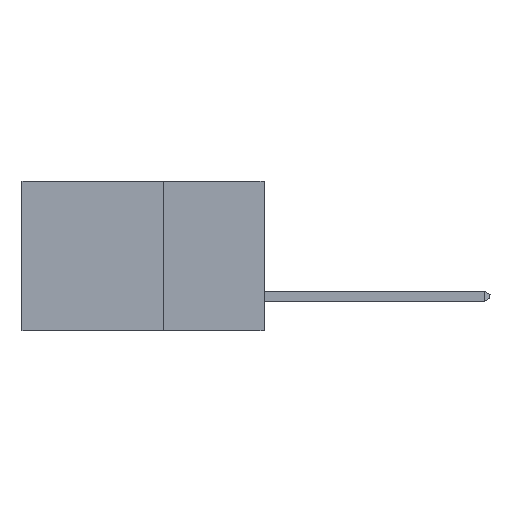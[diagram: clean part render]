
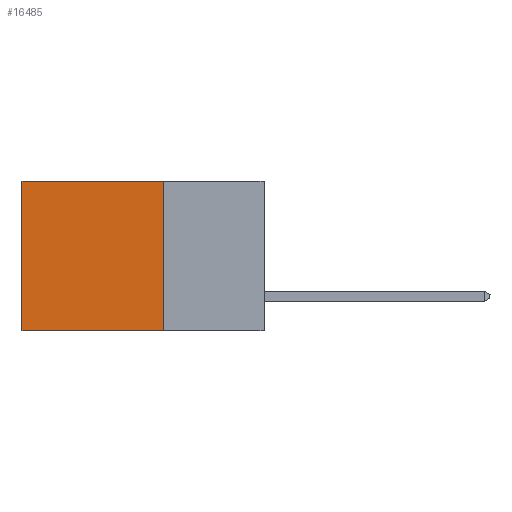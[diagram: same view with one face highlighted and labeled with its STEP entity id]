
A CAD part, left-side view. The second image highlights one B-rep face of the part: STEP entity #16485.
In plain terms, the highlighted planar face has unit normal (-1, 0, 0).
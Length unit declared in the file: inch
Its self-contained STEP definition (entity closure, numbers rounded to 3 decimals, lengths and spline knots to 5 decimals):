
#275 = DIRECTION ( 'NONE',  ( 0., 0., -1. ) ) ;
#851 = CARTESIAN_POINT ( 'NONE',  ( 0.2615, 0.25, -0.37 ) ) ;
#1222 = AXIS2_PLACEMENT_3D ( 'NONE', #851, #7947, #13060 ) ;
#1355 = ORIENTED_EDGE ( 'NONE', *, *, #12639, .T. ) ;
#1738 = DIRECTION ( 'NONE',  ( 0., 1., 0. ) ) ;
#2791 = ORIENTED_EDGE ( 'NONE', *, *, #13741, .T. ) ;
#3584 = LINE ( 'NONE', #10573, #10116 ) ;
#4554 = LINE ( 'NONE', #9725, #14930 ) ;
#5245 = ORIENTED_EDGE ( 'NONE', *, *, #9203, .F. ) ;
#5843 = VERTEX_POINT ( 'NONE', #6564 ) ;
#6564 = CARTESIAN_POINT ( 'NONE',  ( 0.2615, 0.25, 0. ) ) ;
#6592 = VECTOR ( 'NONE', #1738, 39.37008 ) ;
#6628 = VERTEX_POINT ( 'NONE', #19522 ) ;
#6951 = VERTEX_POINT ( 'NONE', #13920 ) ;
#7721 = VECTOR ( 'NONE', #11367, 39.37008 ) ;
#7947 = DIRECTION ( 'NONE',  ( 1., 0., 0. ) ) ;
#9203 = EDGE_CURVE ( 'NONE', #5843, #19078, #3584, .T. ) ;
#9725 = CARTESIAN_POINT ( 'NONE',  ( 0.2615, 0.25, -0.37 ) ) ;
#10116 = VECTOR ( 'NONE', #275, 39.37008 ) ;
#10192 = CARTESIAN_POINT ( 'NONE',  ( 0.2615, 0.25, -0.37 ) ) ;
#10443 = LINE ( 'NONE', #17375, #6592 ) ;
#10573 = CARTESIAN_POINT ( 'NONE',  ( 0.2615, 0.25, -0.37 ) ) ;
#11256 = FACE_OUTER_BOUND ( 'NONE', #16535, .T. ) ;
#11367 = DIRECTION ( 'NONE',  ( 0., 0., -1. ) ) ;
#11544 = EDGE_CURVE ( 'NONE', #19078, #6951, #4554, .T. ) ;
#12639 = EDGE_CURVE ( 'NONE', #5843, #6628, #10443, .T. ) ;
#13060 = DIRECTION ( 'NONE',  ( 0., 0., -1. ) ) ;
#13741 = EDGE_CURVE ( 'NONE', #6628, #6951, #14781, .T. ) ;
#13920 = CARTESIAN_POINT ( 'NONE',  ( 0.2615, 0.6, -0.37 ) ) ;
#14604 = DIRECTION ( 'NONE',  ( 0., 1., 0. ) ) ;
#14781 = LINE ( 'NONE', #18424, #7721 ) ;
#14930 = VECTOR ( 'NONE', #14604, 39.37008 ) ;
#16057 = ORIENTED_EDGE ( 'NONE', *, *, #11544, .F. ) ;
#16478 = PLANE ( 'NONE',  #1222 ) ;
#16485 = ADVANCED_FACE ( 'NONE', ( #11256 ), #16478, .F. ) ;
#16535 = EDGE_LOOP ( 'NONE', ( #2791, #16057, #5245, #1355 ) ) ;
#17375 = CARTESIAN_POINT ( 'NONE',  ( 0.2615, 0.25, 0. ) ) ;
#18424 = CARTESIAN_POINT ( 'NONE',  ( 0.2615, 0.6, -0.37 ) ) ;
#19078 = VERTEX_POINT ( 'NONE', #10192 ) ;
#19522 = CARTESIAN_POINT ( 'NONE',  ( 0.2615, 0.6, 0. ) ) ;
